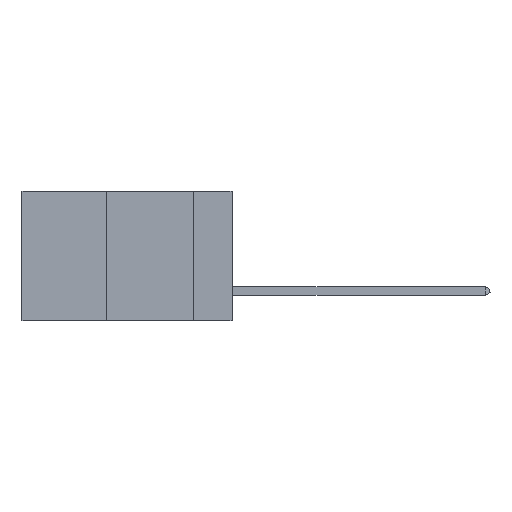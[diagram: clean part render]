
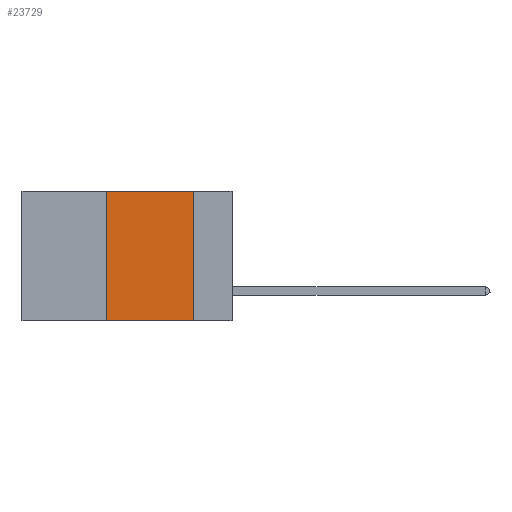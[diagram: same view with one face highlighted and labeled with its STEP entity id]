
A CAD part, left-side view. The second image highlights one B-rep face of the part: STEP entity #23729.
In plain terms, the highlighted planar face has unit normal (-1, 0, 0).
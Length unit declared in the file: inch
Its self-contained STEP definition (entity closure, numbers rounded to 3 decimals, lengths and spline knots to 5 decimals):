
#1464 = VECTOR ( 'NONE', #15013, 39.37008 ) ;
#2577 = EDGE_CURVE ( 'NONE', #8012, #16014, #3494, .T. ) ;
#3494 = LINE ( 'NONE', #4131, #1464 ) ;
#4131 = CARTESIAN_POINT ( 'NONE',  ( 0., 0.6, 0. ) ) ;
#7307 = LINE ( 'NONE', #27729, #21121 ) ;
#7364 = EDGE_CURVE ( 'NONE', #16014, #23659, #11629, .T. ) ;
#7531 = DIRECTION ( 'NONE',  ( 0., 0., -1. ) ) ;
#8012 = VERTEX_POINT ( 'NONE', #25672 ) ;
#8389 = ORIENTED_EDGE ( 'NONE', *, *, #21142, .F. ) ;
#8465 = PLANE ( 'NONE',  #14202 ) ;
#8906 = CARTESIAN_POINT ( 'NONE',  ( 0., 0.36, 0. ) ) ;
#9990 = CARTESIAN_POINT ( 'NONE',  ( 0., 0.11, 0. ) ) ;
#11629 = LINE ( 'NONE', #9990, #21724 ) ;
#12065 = ORIENTED_EDGE ( 'NONE', *, *, #2577, .F. ) ;
#13755 = ORIENTED_EDGE ( 'NONE', *, *, #16669, .T. ) ;
#13901 = VECTOR ( 'NONE', #25872, 39.37008 ) ;
#14202 = AXIS2_PLACEMENT_3D ( 'NONE', #28000, #26159, #21869 ) ;
#14333 = CARTESIAN_POINT ( 'NONE',  ( 0., 0.11, -0.37 ) ) ;
#15013 = DIRECTION ( 'NONE',  ( 0., -1., 0. ) ) ;
#15512 = CARTESIAN_POINT ( 'NONE',  ( 0., 0.11, 0. ) ) ;
#15600 = CARTESIAN_POINT ( 'NONE',  ( 0., 0.36, -0.37 ) ) ;
#16014 = VERTEX_POINT ( 'NONE', #15512 ) ;
#16669 = EDGE_CURVE ( 'NONE', #23418, #23659, #7307, .T. ) ;
#20167 = ORIENTED_EDGE ( 'NONE', *, *, #7364, .F. ) ;
#20839 = FACE_OUTER_BOUND ( 'NONE', #26121, .T. ) ;
#21121 = VECTOR ( 'NONE', #21244, 39.37008 ) ;
#21142 = EDGE_CURVE ( 'NONE', #23418, #8012, #24008, .T. ) ;
#21244 = DIRECTION ( 'NONE',  ( 0., -1., 0. ) ) ;
#21724 = VECTOR ( 'NONE', #7531, 39.37008 ) ;
#21869 = DIRECTION ( 'NONE',  ( 0., 0., -1. ) ) ;
#23418 = VERTEX_POINT ( 'NONE', #15600 ) ;
#23659 = VERTEX_POINT ( 'NONE', #14333 ) ;
#23729 = ADVANCED_FACE ( 'NONE', ( #20839 ), #8465, .F. ) ;
#24008 = LINE ( 'NONE', #8906, #13901 ) ;
#25672 = CARTESIAN_POINT ( 'NONE',  ( 0., 0.36, 0. ) ) ;
#25872 = DIRECTION ( 'NONE',  ( 0., 0., 1. ) ) ;
#26121 = EDGE_LOOP ( 'NONE', ( #20167, #12065, #8389, #13755 ) ) ;
#26159 = DIRECTION ( 'NONE',  ( 1., 0., 0. ) ) ;
#27729 = CARTESIAN_POINT ( 'NONE',  ( 0., 0.6, -0.37 ) ) ;
#28000 = CARTESIAN_POINT ( 'NONE',  ( 0., 0.6, 0. ) ) ;
